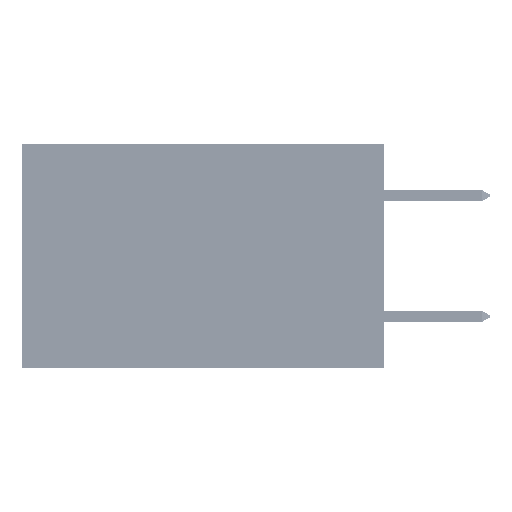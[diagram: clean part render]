
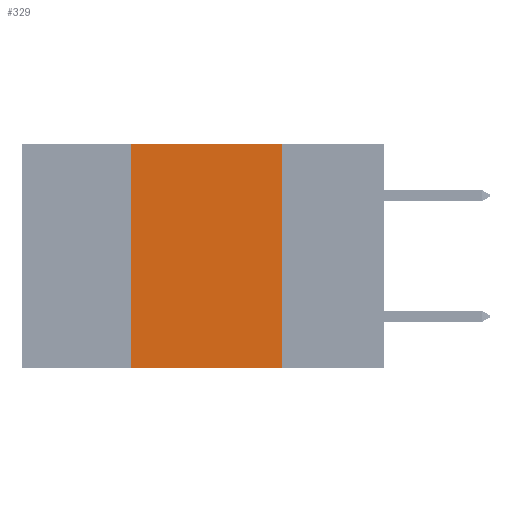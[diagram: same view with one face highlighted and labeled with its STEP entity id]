
A CAD part, left-side view. The second image highlights one B-rep face of the part: STEP entity #329.
In plain terms, the highlighted planar face has unit normal (-1, 0, 0).
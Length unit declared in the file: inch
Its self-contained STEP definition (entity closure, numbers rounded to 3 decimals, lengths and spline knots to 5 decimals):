
#329 = ADVANCED_FACE ( 'NONE', ( #13169 ), #31661, .F. ) ;
#1502 = CARTESIAN_POINT ( 'NONE',  ( 0., 0.17, -0.37 ) ) ;
#2221 = DIRECTION ( 'NONE',  ( 0., 0., -1. ) ) ;
#3325 = DIRECTION ( 'NONE',  ( 0., -1., 0. ) ) ;
#4107 = CARTESIAN_POINT ( 'NONE',  ( 0., 0.42, 0. ) ) ;
#4453 = LINE ( 'NONE', #43832, #23106 ) ;
#5522 = VERTEX_POINT ( 'NONE', #1502 ) ;
#6866 = VECTOR ( 'NONE', #47406, 39.37008 ) ;
#9521 = CARTESIAN_POINT ( 'NONE',  ( 0., 0.42, -0.37 ) ) ;
#10671 = VERTEX_POINT ( 'NONE', #37265 ) ;
#10955 = VECTOR ( 'NONE', #17913, 39.37008 ) ;
#12766 = VERTEX_POINT ( 'NONE', #9521 ) ;
#12896 = EDGE_CURVE ( 'NONE', #12766, #5522, #35943, .T. ) ;
#13169 = FACE_OUTER_BOUND ( 'NONE', #43740, .T. ) ;
#14707 = EDGE_CURVE ( 'NONE', #28086, #10671, #4453, .T. ) ;
#15838 = EDGE_CURVE ( 'NONE', #12766, #28086, #37476, .T. ) ;
#16433 = ORIENTED_EDGE ( 'NONE', *, *, #14707, .F. ) ;
#17913 = DIRECTION ( 'NONE',  ( 0., 0., -1. ) ) ;
#18545 = LINE ( 'NONE', #33335, #10955 ) ;
#18922 = VECTOR ( 'NONE', #42420, 39.37008 ) ;
#19441 = ORIENTED_EDGE ( 'NONE', *, *, #44985, .F. ) ;
#23106 = VECTOR ( 'NONE', #3325, 39.37008 ) ;
#28086 = VERTEX_POINT ( 'NONE', #4107 ) ;
#28383 = DIRECTION ( 'NONE',  ( 1., 0., 0. ) ) ;
#31661 = PLANE ( 'NONE',  #45151 ) ;
#32282 = CARTESIAN_POINT ( 'NONE',  ( 0., 0.6, -0.37 ) ) ;
#33335 = CARTESIAN_POINT ( 'NONE',  ( 0., 0.17, 0. ) ) ;
#35839 = ORIENTED_EDGE ( 'NONE', *, *, #15838, .F. ) ;
#35943 = LINE ( 'NONE', #32282, #6866 ) ;
#36186 = CARTESIAN_POINT ( 'NONE',  ( 0., 0.6, 0. ) ) ;
#37265 = CARTESIAN_POINT ( 'NONE',  ( 0., 0.17, 0. ) ) ;
#37476 = LINE ( 'NONE', #46166, #18922 ) ;
#42004 = ORIENTED_EDGE ( 'NONE', *, *, #12896, .T. ) ;
#42420 = DIRECTION ( 'NONE',  ( 0., 0., 1. ) ) ;
#43740 = EDGE_LOOP ( 'NONE', ( #19441, #16433, #35839, #42004 ) ) ;
#43832 = CARTESIAN_POINT ( 'NONE',  ( 0., 0.6, 0. ) ) ;
#44985 = EDGE_CURVE ( 'NONE', #10671, #5522, #18545, .T. ) ;
#45151 = AXIS2_PLACEMENT_3D ( 'NONE', #36186, #28383, #2221 ) ;
#46166 = CARTESIAN_POINT ( 'NONE',  ( 0., 0.42, 0. ) ) ;
#47406 = DIRECTION ( 'NONE',  ( 0., -1., 0. ) ) ;
